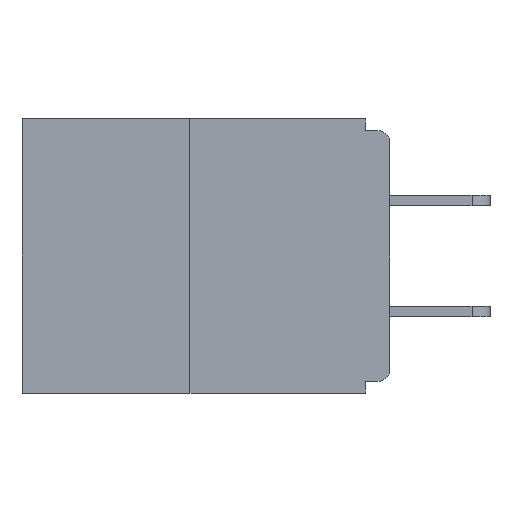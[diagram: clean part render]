
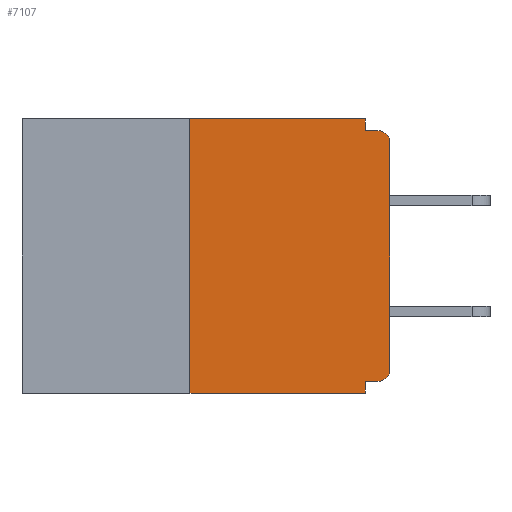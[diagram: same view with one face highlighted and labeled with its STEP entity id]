
A CAD part, left-side view. The second image highlights one B-rep face of the part: STEP entity #7107.
In plain terms, the highlighted planar face has unit normal (-1, 0, 0).
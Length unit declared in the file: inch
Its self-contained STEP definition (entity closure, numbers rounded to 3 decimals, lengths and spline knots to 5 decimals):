
#162 = VECTOR ( 'NONE', #12496, 39.37008 ) ;
#262 = VECTOR ( 'NONE', #13376, 39.37008 ) ;
#718 = DIRECTION ( 'NONE',  ( 0., 1., 0. ) ) ;
#913 = VECTOR ( 'NONE', #718, 39.37008 ) ;
#1025 = DIRECTION ( 'NONE',  ( 0., 0., -1. ) ) ;
#1679 = CARTESIAN_POINT ( 'NONE',  ( 0., 0.031, 0. ) ) ;
#2657 = EDGE_CURVE ( 'NONE', #4438, #11291, #7072, .T. ) ;
#2865 = VECTOR ( 'NONE', #6289, 39.37008 ) ;
#3330 = ORIENTED_EDGE ( 'NONE', *, *, #18276, .F. ) ;
#3349 = DIRECTION ( 'NONE',  ( 0., 0., -1. ) ) ;
#3675 = CARTESIAN_POINT ( 'NONE',  ( 0., 0.031, -0.015 ) ) ;
#3890 = AXIS2_PLACEMENT_3D ( 'NONE', #11135, #9402, #3349 ) ;
#4364 = AXIS2_PLACEMENT_3D ( 'NONE', #13549, #10306, #1025 ) ;
#4438 = VERTEX_POINT ( 'NONE', #1679 ) ;
#4529 = CARTESIAN_POINT ( 'NONE',  ( 0., 0., -0.03 ) ) ;
#4637 = LINE ( 'NONE', #12391, #8047 ) ;
#4973 = LINE ( 'NONE', #14883, #262 ) ;
#4991 = CARTESIAN_POINT ( 'NONE',  ( 0., 0.25, 0. ) ) ;
#5308 = CARTESIAN_POINT ( 'NONE',  ( 0., 0.25, -0.343 ) ) ;
#5639 = AXIS2_PLACEMENT_3D ( 'NONE', #15414, #12259, #7851 ) ;
#5704 = ORIENTED_EDGE ( 'NONE', *, *, #14415, .T. ) ;
#5762 = ORIENTED_EDGE ( 'NONE', *, *, #18923, .T. ) ;
#6218 = CARTESIAN_POINT ( 'NONE',  ( 0., 0.031, 0. ) ) ;
#6289 = DIRECTION ( 'NONE',  ( 0., 0., -1. ) ) ;
#6893 = ORIENTED_EDGE ( 'NONE', *, *, #2657, .F. ) ;
#7072 = LINE ( 'NONE', #6218, #2865 ) ;
#7107 = ADVANCED_FACE ( 'NONE', ( #13221 ), #9473, .F. ) ;
#7787 = LINE ( 'NONE', #13336, #13629 ) ;
#7800 = VERTEX_POINT ( 'NONE', #4991 ) ;
#7851 = DIRECTION ( 'NONE',  ( 0., 0., -1. ) ) ;
#8047 = VECTOR ( 'NONE', #20327, 39.37008 ) ;
#8331 = EDGE_CURVE ( 'NONE', #16419, #10223, #4637, .T. ) ;
#8476 = VERTEX_POINT ( 'NONE', #14246 ) ;
#8526 = ORIENTED_EDGE ( 'NONE', *, *, #8676, .T. ) ;
#8676 = EDGE_CURVE ( 'NONE', #8476, #16770, #7787, .T. ) ;
#8979 = LINE ( 'NONE', #17197, #162 ) ;
#9402 = DIRECTION ( 'NONE',  ( 1., 0., 0. ) ) ;
#9473 = PLANE ( 'NONE',  #3890 ) ;
#9630 = ORIENTED_EDGE ( 'NONE', *, *, #8331, .T. ) ;
#10223 = VERTEX_POINT ( 'NONE', #16578 ) ;
#10306 = DIRECTION ( 'NONE',  ( -1., 0., 0. ) ) ;
#10619 = LINE ( 'NONE', #13501, #19016 ) ;
#11135 = CARTESIAN_POINT ( 'NONE',  ( 0., 0.46, 0. ) ) ;
#11291 = VERTEX_POINT ( 'NONE', #3675 ) ;
#11425 = EDGE_CURVE ( 'NONE', #11291, #12644, #4973, .T. ) ;
#11497 = CARTESIAN_POINT ( 'NONE',  ( 0., 0., -0.328 ) ) ;
#11582 = CARTESIAN_POINT ( 'NONE',  ( 0., 0.031, -0.343 ) ) ;
#11851 = CIRCLE ( 'NONE', #5639, 0.015 ) ;
#12259 = DIRECTION ( 'NONE',  ( -1., 0., 0. ) ) ;
#12382 = DIRECTION ( 'NONE',  ( 0., -1., 0. ) ) ;
#12391 = CARTESIAN_POINT ( 'NONE',  ( 0., 0.46, -0.343 ) ) ;
#12415 = LINE ( 'NONE', #11497, #913 ) ;
#12443 = EDGE_LOOP ( 'NONE', ( #3330, #19859, #9630, #15148, #18057, #5704, #8526, #5762, #14552, #6893 ) ) ;
#12496 = DIRECTION ( 'NONE',  ( 0., 0., 1. ) ) ;
#12542 = LINE ( 'NONE', #11582, #17496 ) ;
#12644 = VERTEX_POINT ( 'NONE', #13908 ) ;
#13161 = VERTEX_POINT ( 'NONE', #18716 ) ;
#13221 = FACE_OUTER_BOUND ( 'NONE', #12443, .T. ) ;
#13336 = CARTESIAN_POINT ( 'NONE',  ( 0., 0., 0. ) ) ;
#13376 = DIRECTION ( 'NONE',  ( 0., -1., 0. ) ) ;
#13480 = EDGE_CURVE ( 'NONE', #13161, #20159, #12415, .T. ) ;
#13501 = CARTESIAN_POINT ( 'NONE',  ( 0., 0.46, 0. ) ) ;
#13549 = CARTESIAN_POINT ( 'NONE',  ( 0., 0.015, -0.313 ) ) ;
#13629 = VECTOR ( 'NONE', #19817, 39.37008 ) ;
#13908 = CARTESIAN_POINT ( 'NONE',  ( 0., 0.015, -0.015 ) ) ;
#14246 = CARTESIAN_POINT ( 'NONE',  ( 0., 0., -0.313 ) ) ;
#14415 = EDGE_CURVE ( 'NONE', #13161, #8476, #18055, .T. ) ;
#14552 = ORIENTED_EDGE ( 'NONE', *, *, #11425, .F. ) ;
#14720 = DIRECTION ( 'NONE',  ( 0., 0., -1. ) ) ;
#14883 = CARTESIAN_POINT ( 'NONE',  ( 0., 0., -0.015 ) ) ;
#15148 = ORIENTED_EDGE ( 'NONE', *, *, #19445, .F. ) ;
#15414 = CARTESIAN_POINT ( 'NONE',  ( 0., 0.015, -0.03 ) ) ;
#15908 = CARTESIAN_POINT ( 'NONE',  ( 0., 0.031, -0.328 ) ) ;
#16419 = VERTEX_POINT ( 'NONE', #5308 ) ;
#16578 = CARTESIAN_POINT ( 'NONE',  ( 0., 0.031, -0.343 ) ) ;
#16769 = EDGE_CURVE ( 'NONE', #16419, #7800, #8979, .T. ) ;
#16770 = VERTEX_POINT ( 'NONE', #4529 ) ;
#17197 = CARTESIAN_POINT ( 'NONE',  ( 0., 0.25, 0. ) ) ;
#17496 = VECTOR ( 'NONE', #14720, 39.37008 ) ;
#18055 = CIRCLE ( 'NONE', #4364, 0.015 ) ;
#18057 = ORIENTED_EDGE ( 'NONE', *, *, #13480, .F. ) ;
#18276 = EDGE_CURVE ( 'NONE', #7800, #4438, #10619, .T. ) ;
#18716 = CARTESIAN_POINT ( 'NONE',  ( 0., 0.015, -0.328 ) ) ;
#18923 = EDGE_CURVE ( 'NONE', #16770, #12644, #11851, .T. ) ;
#19016 = VECTOR ( 'NONE', #12382, 39.37008 ) ;
#19445 = EDGE_CURVE ( 'NONE', #20159, #10223, #12542, .T. ) ;
#19817 = DIRECTION ( 'NONE',  ( 0., 0., 1. ) ) ;
#19859 = ORIENTED_EDGE ( 'NONE', *, *, #16769, .F. ) ;
#20159 = VERTEX_POINT ( 'NONE', #15908 ) ;
#20327 = DIRECTION ( 'NONE',  ( 0., -1., 0. ) ) ;
